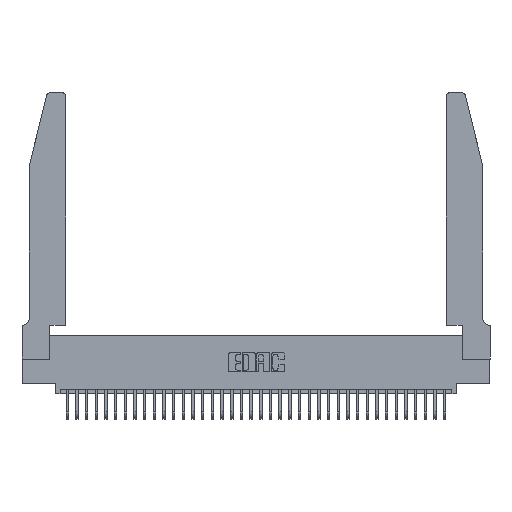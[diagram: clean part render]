
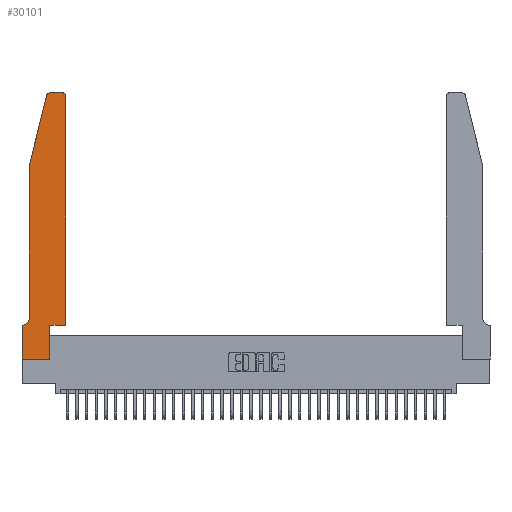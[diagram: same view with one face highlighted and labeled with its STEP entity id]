
A CAD part, top view. The second image highlights one B-rep face of the part: STEP entity #30101.
In plain terms, the highlighted planar face has unit normal (0, 0, 1).
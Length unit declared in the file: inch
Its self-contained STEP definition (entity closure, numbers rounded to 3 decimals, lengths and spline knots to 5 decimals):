
#17 = DIRECTION ( 'NONE',  ( 0., 0., 1. ) ) ;
#272 = CARTESIAN_POINT ( 'NONE',  ( 0.284, 2.75, 0.37 ) ) ;
#811 = AXIS2_PLACEMENT_3D ( 'NONE', #18024, #17, #20962 ) ;
#836 = DIRECTION ( 'NONE',  ( 1., 0., 0. ) ) ;
#1871 = CARTESIAN_POINT ( 'NONE',  ( 0., 0., 0.37 ) ) ;
#2319 = CARTESIAN_POINT ( 'NONE',  ( 0.4505, 2.72, 0.37 ) ) ;
#2834 = VERTEX_POINT ( 'NONE', #37622 ) ;
#3068 = CARTESIAN_POINT ( 'NONE',  ( 0.25487, 2.72718, 0.37 ) ) ;
#3454 = VECTOR ( 'NONE', #16097, 39.37008 ) ;
#3657 = VECTOR ( 'NONE', #16983, 39.37008 ) ;
#3839 = CARTESIAN_POINT ( 'NONE',  ( 0.4505, 0.35, 0.37 ) ) ;
#4269 = ORIENTED_EDGE ( 'NONE', *, *, #17762, .T. ) ;
#5682 = VECTOR ( 'NONE', #22736, 39.37008 ) ;
#5704 = CARTESIAN_POINT ( 'NONE',  ( 0.2605, 2.75, 0.37 ) ) ;
#6035 = CIRCLE ( 'NONE', #811, 0.03 ) ;
#6653 = CARTESIAN_POINT ( 'NONE',  ( 0.4505, 0.35, 0.37 ) ) ;
#6676 = DIRECTION ( 'NONE',  ( 0., 0., -1. ) ) ;
#7470 = VERTEX_POINT ( 'NONE', #272 ) ;
#7551 = ORIENTED_EDGE ( 'NONE', *, *, #34347, .T. ) ;
#8044 = ORIENTED_EDGE ( 'NONE', *, *, #26778, .T. ) ;
#8050 = AXIS2_PLACEMENT_3D ( 'NONE', #8598, #29188, #11636 ) ;
#8500 = DIRECTION ( 'NONE',  ( 0., 1., 0. ) ) ;
#8596 = VERTEX_POINT ( 'NONE', #2319 ) ;
#8598 = CARTESIAN_POINT ( 'NONE',  ( 0.4205, 2.72, 0.37 ) ) ;
#8814 = VECTOR ( 'NONE', #32831, 39.37008 ) ;
#9193 = LINE ( 'NONE', #29472, #23079 ) ;
#9718 = VERTEX_POINT ( 'NONE', #12136 ) ;
#9904 = VECTOR ( 'NONE', #24365, 39.37008 ) ;
#10526 = LINE ( 'NONE', #33533, #3454 ) ;
#11128 = EDGE_CURVE ( 'NONE', #9718, #27372, #22423, .T. ) ;
#11403 = VERTEX_POINT ( 'NONE', #3068 ) ;
#11636 = DIRECTION ( 'NONE',  ( 1., 0., 0. ) ) ;
#12136 = CARTESIAN_POINT ( 'NONE',  ( 0., 0.35, 0.37 ) ) ;
#12598 = LINE ( 'NONE', #13986, #3657 ) ;
#12716 = ORIENTED_EDGE ( 'NONE', *, *, #36062, .T. ) ;
#13229 = LINE ( 'NONE', #23259, #18338 ) ;
#13792 = CARTESIAN_POINT ( 'NONE',  ( 0., 0.35, 0.37 ) ) ;
#13923 = DIRECTION ( 'NONE',  ( 1., 0., 0. ) ) ;
#13986 = CARTESIAN_POINT ( 'NONE',  ( 0.0755, 2., 0.37 ) ) ;
#14451 = EDGE_CURVE ( 'NONE', #23562, #9718, #9193, .T. ) ;
#15130 = AXIS2_PLACEMENT_3D ( 'NONE', #24391, #6676, #27320 ) ;
#16097 = DIRECTION ( 'NONE',  ( 1., 0., 0. ) ) ;
#16676 = EDGE_CURVE ( 'NONE', #23533, #29874, #10526, .T. ) ;
#16983 = DIRECTION ( 'NONE',  ( 0., -1., 0. ) ) ;
#17392 = ORIENTED_EDGE ( 'NONE', *, *, #28225, .T. ) ;
#17469 = VERTEX_POINT ( 'NONE', #28979 ) ;
#17493 = VERTEX_POINT ( 'NONE', #17540 ) ;
#17540 = CARTESIAN_POINT ( 'NONE',  ( 0.2865, 0., 0.37 ) ) ;
#17762 = EDGE_CURVE ( 'NONE', #27372, #17493, #29779, .T. ) ;
#18024 = CARTESIAN_POINT ( 'NONE',  ( 0.284, 2.72, 0.37 ) ) ;
#18338 = VECTOR ( 'NONE', #8500, 39.37008 ) ;
#19697 = CARTESIAN_POINT ( 'NONE',  ( 0.2865, 0.35, 0.37 ) ) ;
#19730 = PLANE ( 'NONE',  #23243 ) ;
#20069 = LINE ( 'NONE', #5704, #34614 ) ;
#20447 = EDGE_CURVE ( 'NONE', #7470, #11403, #6035, .T. ) ;
#20884 = VERTEX_POINT ( 'NONE', #37162 ) ;
#20962 = DIRECTION ( 'NONE',  ( 1., 0., 0. ) ) ;
#22403 = ORIENTED_EDGE ( 'NONE', *, *, #27542, .T. ) ;
#22423 = LINE ( 'NONE', #1871, #5682 ) ;
#22736 = DIRECTION ( 'NONE',  ( 0., -1., 0. ) ) ;
#22866 = EDGE_LOOP ( 'NONE', ( #12716, #36924, #22403, #7551, #17392, #32845, #26942, #4269, #28761, #36493, #30595, #8044 ) ) ;
#23079 = VECTOR ( 'NONE', #35306, 39.37008 ) ;
#23243 = AXIS2_PLACEMENT_3D ( 'NONE', #13792, #31431, #13923 ) ;
#23259 = CARTESIAN_POINT ( 'NONE',  ( 0.2865, 0.35, 0.37 ) ) ;
#23533 = VERTEX_POINT ( 'NONE', #19697 ) ;
#23562 = VERTEX_POINT ( 'NONE', #25516 ) ;
#24365 = DIRECTION ( 'NONE',  ( 0., 1., 0. ) ) ;
#24391 = CARTESIAN_POINT ( 'NONE',  ( 0.0055, 0.42, 0.37 ) ) ;
#24402 = FACE_OUTER_BOUND ( 'NONE', #22866, .T. ) ;
#25420 = EDGE_CURVE ( 'NONE', #17493, #23533, #13229, .T. ) ;
#25423 = LINE ( 'NONE', #29915, #8814 ) ;
#25516 = CARTESIAN_POINT ( 'NONE',  ( 0.0055, 0.35, 0.37 ) ) ;
#25560 = LINE ( 'NONE', #6653, #9904 ) ;
#25698 = EDGE_CURVE ( 'NONE', #29874, #8596, #25560, .T. ) ;
#26363 = CARTESIAN_POINT ( 'NONE',  ( 0., 0., 0.37 ) ) ;
#26392 = DIRECTION ( 'NONE',  ( -1., 0., 0. ) ) ;
#26772 = CIRCLE ( 'NONE', #15130, 0.07 ) ;
#26778 = EDGE_CURVE ( 'NONE', #8596, #2834, #34583, .T. ) ;
#26942 = ORIENTED_EDGE ( 'NONE', *, *, #11128, .T. ) ;
#27320 = DIRECTION ( 'NONE',  ( -1., 0., 0. ) ) ;
#27372 = VERTEX_POINT ( 'NONE', #26363 ) ;
#27542 = EDGE_CURVE ( 'NONE', #11403, #17469, #25423, .T. ) ;
#28225 = EDGE_CURVE ( 'NONE', #20884, #23562, #26772, .T. ) ;
#28761 = ORIENTED_EDGE ( 'NONE', *, *, #25420, .T. ) ;
#28979 = CARTESIAN_POINT ( 'NONE',  ( 0.0755, 2., 0.37 ) ) ;
#29188 = DIRECTION ( 'NONE',  ( 0., 0., 1. ) ) ;
#29472 = CARTESIAN_POINT ( 'NONE',  ( 0.0755, 0.35, 0.37 ) ) ;
#29779 = LINE ( 'NONE', #33278, #36598 ) ;
#29874 = VERTEX_POINT ( 'NONE', #3839 ) ;
#29915 = CARTESIAN_POINT ( 'NONE',  ( 0.0755, 2., 0.37 ) ) ;
#30101 = ADVANCED_FACE ( 'NONE', ( #24402 ), #19730, .T. ) ;
#30595 = ORIENTED_EDGE ( 'NONE', *, *, #25698, .T. ) ;
#31431 = DIRECTION ( 'NONE',  ( 0., 0., 1. ) ) ;
#32831 = DIRECTION ( 'NONE',  ( -0.239, -0.971, 0. ) ) ;
#32845 = ORIENTED_EDGE ( 'NONE', *, *, #14451, .T. ) ;
#33278 = CARTESIAN_POINT ( 'NONE',  ( 0., 0., 0.37 ) ) ;
#33533 = CARTESIAN_POINT ( 'NONE',  ( 0.4505, 0.35, 0.37 ) ) ;
#34347 = EDGE_CURVE ( 'NONE', #17469, #20884, #12598, .T. ) ;
#34583 = CIRCLE ( 'NONE', #8050, 0.03 ) ;
#34614 = VECTOR ( 'NONE', #26392, 39.37008 ) ;
#35306 = DIRECTION ( 'NONE',  ( -1., 0., 0. ) ) ;
#36062 = EDGE_CURVE ( 'NONE', #2834, #7470, #20069, .T. ) ;
#36493 = ORIENTED_EDGE ( 'NONE', *, *, #16676, .T. ) ;
#36598 = VECTOR ( 'NONE', #836, 39.37008 ) ;
#36924 = ORIENTED_EDGE ( 'NONE', *, *, #20447, .T. ) ;
#37162 = CARTESIAN_POINT ( 'NONE',  ( 0.0755, 0.42, 0.37 ) ) ;
#37622 = CARTESIAN_POINT ( 'NONE',  ( 0.4205, 2.75, 0.37 ) ) ;
